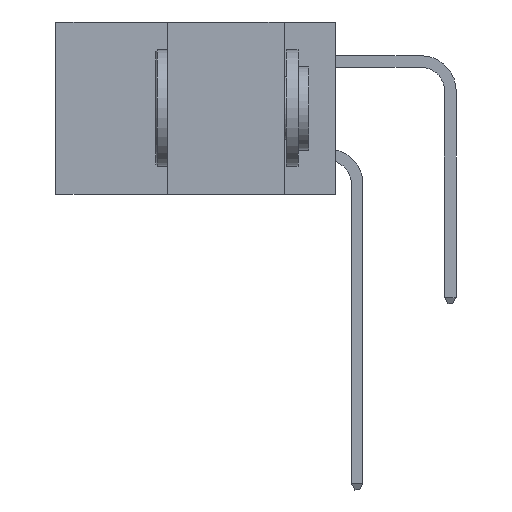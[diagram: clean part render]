
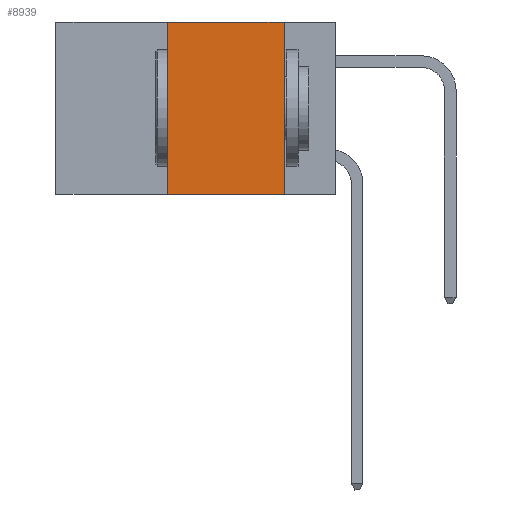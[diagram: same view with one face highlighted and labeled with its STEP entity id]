
A CAD part, left-side view. The second image highlights one B-rep face of the part: STEP entity #8939.
In plain terms, the highlighted planar face has unit normal (-1, 0, 0).
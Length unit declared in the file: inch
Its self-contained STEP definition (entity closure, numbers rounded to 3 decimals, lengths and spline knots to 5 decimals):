
#689 = ORIENTED_EDGE ( 'NONE', *, *, #22936, .F. ) ;
#845 = VECTOR ( 'NONE', #17039, 39.37008 ) ;
#863 = ORIENTED_EDGE ( 'NONE', *, *, #3251, .T. ) ;
#2548 = EDGE_CURVE ( 'NONE', #5544, #11459, #17119, .T. ) ;
#3251 = EDGE_CURVE ( 'NONE', #7275, #26624, #11267, .T. ) ;
#5478 = CARTESIAN_POINT ( 'NONE',  ( 0., 0.36, 0. ) ) ;
#5544 = VERTEX_POINT ( 'NONE', #5478 ) ;
#5671 = DIRECTION ( 'NONE',  ( 0., 0., 1. ) ) ;
#6704 = CARTESIAN_POINT ( 'NONE',  ( 0., 0.11, -0.37 ) ) ;
#7275 = VERTEX_POINT ( 'NONE', #13806 ) ;
#8483 = CARTESIAN_POINT ( 'NONE',  ( 0., 0.6, -0.37 ) ) ;
#8873 = DIRECTION ( 'NONE',  ( 0., 0., -1. ) ) ;
#8939 = ADVANCED_FACE ( 'NONE', ( #19517 ), #21373, .F. ) ;
#10334 = AXIS2_PLACEMENT_3D ( 'NONE', #15329, #25714, #8873 ) ;
#10966 = EDGE_CURVE ( 'NONE', #11459, #26624, #14277, .T. ) ;
#11267 = LINE ( 'NONE', #8483, #21326 ) ;
#11459 = VERTEX_POINT ( 'NONE', #13756 ) ;
#13576 = CARTESIAN_POINT ( 'NONE',  ( 0., 0.6, 0. ) ) ;
#13756 = CARTESIAN_POINT ( 'NONE',  ( 0., 0.11, 0. ) ) ;
#13806 = CARTESIAN_POINT ( 'NONE',  ( 0., 0.36, -0.37 ) ) ;
#13994 = ORIENTED_EDGE ( 'NONE', *, *, #10966, .F. ) ;
#13993 = CARTESIAN_POINT ( 'NONE',  ( 0., 0.36, 0. ) ) ;
#14277 = LINE ( 'NONE', #16318, #845 ) ;
#15329 = CARTESIAN_POINT ( 'NONE',  ( 0., 0.6, 0. ) ) ;
#16318 = CARTESIAN_POINT ( 'NONE',  ( 0., 0.11, 0. ) ) ;
#16372 = DIRECTION ( 'NONE',  ( 0., -1., 0. ) ) ;
#16866 = DIRECTION ( 'NONE',  ( 0., -1., 0. ) ) ;
#17039 = DIRECTION ( 'NONE',  ( 0., 0., -1. ) ) ;
#17119 = LINE ( 'NONE', #13576, #23644 ) ;
#17320 = ORIENTED_EDGE ( 'NONE', *, *, #2548, .F. ) ;
#19517 = FACE_OUTER_BOUND ( 'NONE', #22903, .T. ) ;
#21326 = VECTOR ( 'NONE', #16866, 39.37008 ) ;
#21373 = PLANE ( 'NONE',  #10334 ) ;
#21797 = VECTOR ( 'NONE', #5671, 39.37008 ) ;
#22112 = LINE ( 'NONE', #13993, #21797 ) ;
#22903 = EDGE_LOOP ( 'NONE', ( #13994, #17320, #689, #863 ) ) ;
#22936 = EDGE_CURVE ( 'NONE', #7275, #5544, #22112, .T. ) ;
#23644 = VECTOR ( 'NONE', #16372, 39.37008 ) ;
#25714 = DIRECTION ( 'NONE',  ( 1., 0., 0. ) ) ;
#26624 = VERTEX_POINT ( 'NONE', #6704 ) ;
